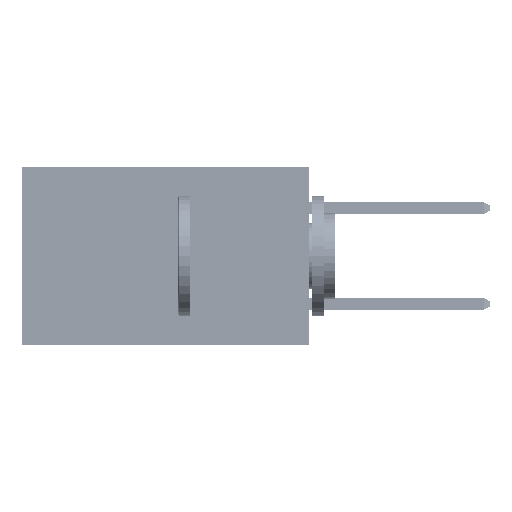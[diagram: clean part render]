
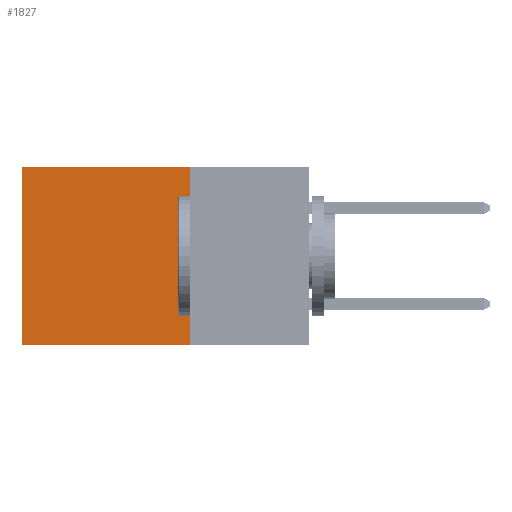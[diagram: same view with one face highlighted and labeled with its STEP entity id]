
A CAD part, left-side view. The second image highlights one B-rep face of the part: STEP entity #1827.
In plain terms, the highlighted planar face has unit normal (-1, 0, 0).
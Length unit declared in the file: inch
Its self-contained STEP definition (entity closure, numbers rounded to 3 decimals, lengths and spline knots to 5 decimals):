
#572 = DIRECTION ( 'NONE',  ( 0., 0., -1. ) ) ;
#826 = VERTEX_POINT ( 'NONE', #5717 ) ;
#1252 = ORIENTED_EDGE ( 'NONE', *, *, #6919, .F. ) ;
#1253 = EDGE_CURVE ( 'NONE', #29932, #826, #50487, .T. ) ;
#1827 = ADVANCED_FACE ( 'NONE', ( #39785 ), #15815, .F. ) ;
#2955 = VERTEX_POINT ( 'NONE', #47054 ) ;
#3040 = ORIENTED_EDGE ( 'NONE', *, *, #17949, .F. ) ;
#3041 = LINE ( 'NONE', #14914, #4282 ) ;
#4282 = VECTOR ( 'NONE', #26785, 39.37008 ) ;
#4986 = VECTOR ( 'NONE', #51725, 39.37008 ) ;
#5717 = CARTESIAN_POINT ( 'NONE',  ( 0.2875, 0.6, -0.37 ) ) ;
#6919 = EDGE_CURVE ( 'NONE', #44598, #826, #48880, .T. ) ;
#8326 = CARTESIAN_POINT ( 'NONE',  ( 0.2875, 0.6, 0. ) ) ;
#14914 = CARTESIAN_POINT ( 'NONE',  ( 0.2875, 0.25, 0. ) ) ;
#15815 = PLANE ( 'NONE',  #20407 ) ;
#17949 = EDGE_CURVE ( 'NONE', #2955, #44598, #48815, .T. ) ;
#19436 = ORIENTED_EDGE ( 'NONE', *, *, #1253, .T. ) ;
#20407 = AXIS2_PLACEMENT_3D ( 'NONE', #39319, #39674, #35445 ) ;
#21832 = ORIENTED_EDGE ( 'NONE', *, *, #39177, .T. ) ;
#22952 = CARTESIAN_POINT ( 'NONE',  ( 0.2875, 0.6, 0. ) ) ;
#24413 = DIRECTION ( 'NONE',  ( 0., 0., -1. ) ) ;
#26785 = DIRECTION ( 'NONE',  ( 0., 1., 0. ) ) ;
#27529 = CARTESIAN_POINT ( 'NONE',  ( 0.2875, 0.25, -0.37 ) ) ;
#29932 = VERTEX_POINT ( 'NONE', #22952 ) ;
#32257 = CARTESIAN_POINT ( 'NONE',  ( 0.2875, 0.25, -0.37 ) ) ;
#32545 = VECTOR ( 'NONE', #572, 39.37008 ) ;
#35445 = DIRECTION ( 'NONE',  ( 0., 0., -1. ) ) ;
#39177 = EDGE_CURVE ( 'NONE', #2955, #29932, #3041, .T. ) ;
#39319 = CARTESIAN_POINT ( 'NONE',  ( 0.2875, 0.25, 0. ) ) ;
#39674 = DIRECTION ( 'NONE',  ( 1., 0., 0. ) ) ;
#39785 = FACE_OUTER_BOUND ( 'NONE', #49459, .T. ) ;
#41051 = CARTESIAN_POINT ( 'NONE',  ( 0.2875, 0.25, 0. ) ) ;
#44598 = VERTEX_POINT ( 'NONE', #32257 ) ;
#47054 = CARTESIAN_POINT ( 'NONE',  ( 0.2875, 0.25, 0. ) ) ;
#48815 = LINE ( 'NONE', #41051, #32545 ) ;
#48880 = LINE ( 'NONE', #27529, #4986 ) ;
#49235 = VECTOR ( 'NONE', #24413, 39.37008 ) ;
#49459 = EDGE_LOOP ( 'NONE', ( #19436, #1252, #3040, #21832 ) ) ;
#50487 = LINE ( 'NONE', #8326, #49235 ) ;
#51725 = DIRECTION ( 'NONE',  ( 0., 1., 0. ) ) ;
